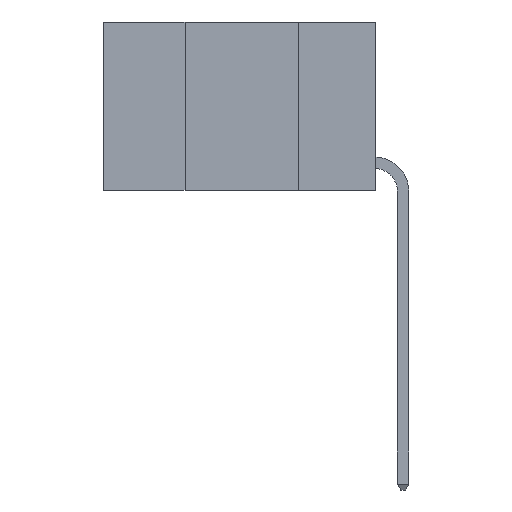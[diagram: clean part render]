
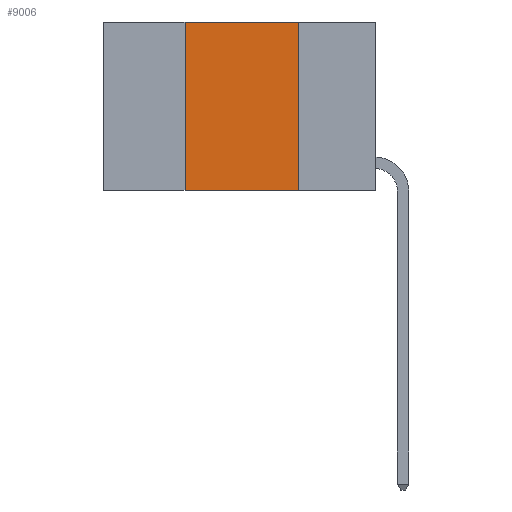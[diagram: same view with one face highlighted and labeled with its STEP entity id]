
A CAD part, left-side view. The second image highlights one B-rep face of the part: STEP entity #9006.
In plain terms, the highlighted planar face has unit normal (-1, 0, 0).
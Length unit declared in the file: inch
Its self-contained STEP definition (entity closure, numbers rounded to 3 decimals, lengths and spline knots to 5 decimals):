
#687 = CARTESIAN_POINT ( 'NONE',  ( 0., 0.42, 0. ) ) ;
#781 = ORIENTED_EDGE ( 'NONE', *, *, #9324, .F. ) ;
#1474 = DIRECTION ( 'NONE',  ( 0., 0., 1. ) ) ;
#1490 = VECTOR ( 'NONE', #3607, 39.37008 ) ;
#1753 = ORIENTED_EDGE ( 'NONE', *, *, #8644, .T. ) ;
#1891 = EDGE_LOOP ( 'NONE', ( #5034, #5210, #781, #1753 ) ) ;
#1939 = VECTOR ( 'NONE', #2248, 39.37008 ) ;
#2050 = VECTOR ( 'NONE', #1474, 39.37008 ) ;
#2248 = DIRECTION ( 'NONE',  ( 0., -1., 0. ) ) ;
#2300 = EDGE_CURVE ( 'NONE', #6830, #2631, #3526, .T. ) ;
#2381 = VECTOR ( 'NONE', #8578, 39.37008 ) ;
#2631 = VERTEX_POINT ( 'NONE', #5469 ) ;
#3526 = LINE ( 'NONE', #8483, #2381 ) ;
#3607 = DIRECTION ( 'NONE',  ( 0., 0., -1. ) ) ;
#3660 = LINE ( 'NONE', #9623, #1490 ) ;
#3830 = VERTEX_POINT ( 'NONE', #5220 ) ;
#4313 = EDGE_CURVE ( 'NONE', #2631, #4335, #3660, .T. ) ;
#4318 = CARTESIAN_POINT ( 'NONE',  ( 0., 0.6, 0. ) ) ;
#4335 = VERTEX_POINT ( 'NONE', #8895 ) ;
#5034 = ORIENTED_EDGE ( 'NONE', *, *, #4313, .F. ) ;
#5078 = DIRECTION ( 'NONE',  ( 0., 0., -1. ) ) ;
#5210 = ORIENTED_EDGE ( 'NONE', *, *, #2300, .F. ) ;
#5220 = CARTESIAN_POINT ( 'NONE',  ( 0., 0.42, -0.37 ) ) ;
#5400 = CARTESIAN_POINT ( 'NONE',  ( 0., 0.6, -0.37 ) ) ;
#5469 = CARTESIAN_POINT ( 'NONE',  ( 0., 0.17, 0. ) ) ;
#6141 = LINE ( 'NONE', #5400, #1939 ) ;
#6830 = VERTEX_POINT ( 'NONE', #687 ) ;
#8115 = PLANE ( 'NONE',  #8959 ) ;
#8220 = LINE ( 'NONE', #9181, #2050 ) ;
#8483 = CARTESIAN_POINT ( 'NONE',  ( 0., 0.6, 0. ) ) ;
#8578 = DIRECTION ( 'NONE',  ( 0., -1., 0. ) ) ;
#8583 = FACE_OUTER_BOUND ( 'NONE', #1891, .T. ) ;
#8644 = EDGE_CURVE ( 'NONE', #3830, #4335, #6141, .T. ) ;
#8895 = CARTESIAN_POINT ( 'NONE',  ( 0., 0.17, -0.37 ) ) ;
#8959 = AXIS2_PLACEMENT_3D ( 'NONE', #4318, #9600, #5078 ) ;
#9006 = ADVANCED_FACE ( 'NONE', ( #8583 ), #8115, .F. ) ;
#9181 = CARTESIAN_POINT ( 'NONE',  ( 0., 0.42, 0. ) ) ;
#9324 = EDGE_CURVE ( 'NONE', #3830, #6830, #8220, .T. ) ;
#9600 = DIRECTION ( 'NONE',  ( 1., 0., 0. ) ) ;
#9623 = CARTESIAN_POINT ( 'NONE',  ( 0., 0.17, 0. ) ) ;
